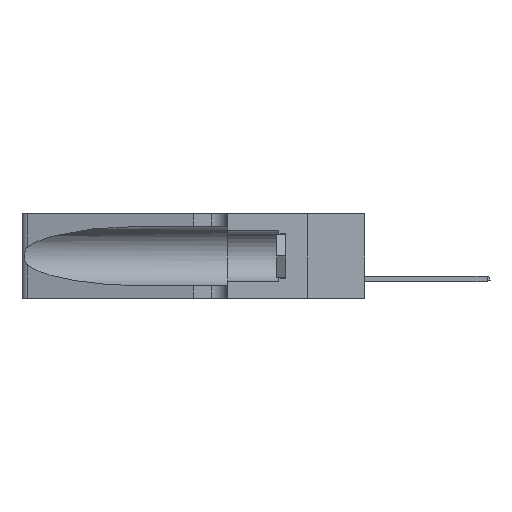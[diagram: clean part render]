
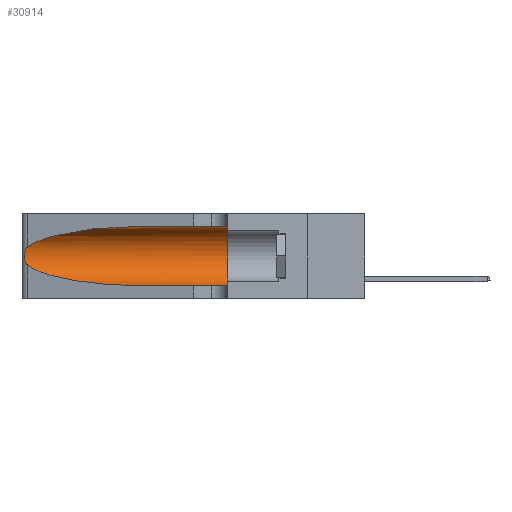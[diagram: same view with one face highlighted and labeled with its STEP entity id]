
A CAD part, left-side view. The second image highlights one B-rep face of the part: STEP entity #30914.
In plain terms, the highlighted cylindrical face has radius 3.308 mm (diameter 6.617 mm), a partial arc.
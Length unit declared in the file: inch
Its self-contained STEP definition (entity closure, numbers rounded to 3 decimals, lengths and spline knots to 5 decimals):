
#700 = CARTESIAN_POINT ( 'NONE',  ( 0.1305, 1.61858, 0.185 ) ) ;
#908 = CARTESIAN_POINT ( 'NONE',  ( 0.2373, 1.15595, 0.08982 ) ) ;
#1054 = ORIENTED_EDGE ( 'NONE', *, *, #3222, .T. ) ;
#1078 = CARTESIAN_POINT ( 'NONE',  ( 0.25487, 1.22718, 0.22369 ) ) ;
#1785 = CARTESIAN_POINT ( 'NONE',  ( 0.26017, 1.23833, 0.17102 ) ) ;
#2062 = CARTESIAN_POINT ( 'NONE',  ( 0.25555, 1.22993, 0.14849 ) ) ;
#3222 = EDGE_CURVE ( 'NONE', #4837, #20518, #38762, .T. ) ;
#4233 = DIRECTION ( 'NONE',  ( 0., -1., 0. ) ) ;
#4286 = CARTESIAN_POINT ( 'NONE',  ( 0.1305, 1.61858, 0.31525 ) ) ;
#4837 = VERTEX_POINT ( 'NONE', #37128 ) ;
#4975 = LINE ( 'NONE', #4286, #26247 ) ;
#5872 = ORIENTED_EDGE ( 'NONE', *, *, #35247, .F. ) ;
#5877 = FACE_OUTER_BOUND ( 'NONE', #23993, .T. ) ;
#6115 = AXIS2_PLACEMENT_3D ( 'NONE', #31212, #37541, #15209 ) ;
#6388 = ORIENTED_EDGE ( 'NONE', *, *, #33840, .F. ) ;
#6869 = CARTESIAN_POINT ( 'NONE',  ( 0.25487, 1.22718, 0.14631 ) ) ;
#7342 = CARTESIAN_POINT ( 'NONE',  ( 0.18966, 0.96281, 0.31525 ) ) ;
#7866 = VERTEX_POINT ( 'NONE', #13988 ) ;
#8295 = CARTESIAN_POINT ( 'NONE',  ( 0.25487, 1.22718, 0.14631 ) ) ;
#9068 = CARTESIAN_POINT ( 'NONE',  ( 0.1305, 0.72297, 0.31525 ) ) ;
#9539 = CARTESIAN_POINT ( 'NONE',  ( 0.1305, 0.35, 0.31525 ) ) ;
#9937 =( BOUNDED_CURVE ( )  B_SPLINE_CURVE ( 3, ( #9068, #7342, #10147, #1078 ),
 .UNSPECIFIED., .F., .F. ) 
 B_SPLINE_CURVE_WITH_KNOTS ( ( 4, 4 ),
 ( 1.5708, 2.84003 ),
 .UNSPECIFIED. ) 
 CURVE ( )  GEOMETRIC_REPRESENTATION_ITEM ( )  RATIONAL_B_SPLINE_CURVE ( ( 1., 0.87, 0.87, 1. ) ) 
 REPRESENTATION_ITEM ( '' )  );
#10120 = CARTESIAN_POINT ( 'NONE',  ( 0.18966, 0.96281, 0.05475 ) ) ;
#10147 = CARTESIAN_POINT ( 'NONE',  ( 0.2373, 1.15595, 0.28018 ) ) ;
#11411 = CARTESIAN_POINT ( 'NONE',  ( 0.25787, 1.23484, 0.2124 ) ) ;
#12643 = ORIENTED_EDGE ( 'NONE', *, *, #15343, .T. ) ;
#13561 = DIRECTION ( 'NONE',  ( 0., 0., -1. ) ) ;
#13988 = CARTESIAN_POINT ( 'NONE',  ( 0.1305, 0.72297, 0.31525 ) ) ;
#14921 = CARTESIAN_POINT ( 'NONE',  ( 0.25854, 1.2359, 0.20912 ) ) ;
#15205 = CARTESIAN_POINT ( 'NONE',  ( 0.26075, 1.23896, 0.178 ) ) ;
#15209 = DIRECTION ( 'NONE',  ( 0., 0., 1. ) ) ;
#15343 = EDGE_CURVE ( 'NONE', #7866, #41217, #9937, .T. ) ;
#20518 = VERTEX_POINT ( 'NONE', #26975 ) ;
#21016 = CARTESIAN_POINT ( 'NONE',  ( 0.25856, 1.23593, 0.16098 ) ) ;
#21431 = CARTESIAN_POINT ( 'NONE',  ( 0.25639, 1.23186, 0.15144 ) ) ;
#21580 = CARTESIAN_POINT ( 'NONE',  ( 0.25487, 1.22718, 0.22369 ) ) ;
#22164 = VERTEX_POINT ( 'NONE', #25880 ) ;
#23993 = EDGE_LOOP ( 'NONE', ( #12643, #41035, #24847, #1054, #5872, #6388 ) ) ;
#24411 = CARTESIAN_POINT ( 'NONE',  ( 0.25789, 1.23486, 0.15765 ) ) ;
#24847 = ORIENTED_EDGE ( 'NONE', *, *, #32039, .T. ) ;
#25765 = DIRECTION ( 'NONE',  ( 0., -1., 0. ) ) ;
#25880 = CARTESIAN_POINT ( 'NONE',  ( 0.25487, 1.22718, 0.14631 ) ) ;
#26092 = CARTESIAN_POINT ( 'NONE',  ( 0.1305, 0.72297, 0.05475 ) ) ;
#26247 = VECTOR ( 'NONE', #30467, 39.37008 ) ;
#26975 = CARTESIAN_POINT ( 'NONE',  ( 0.1305, 0.35, 0.05475 ) ) ;
#27406 =( BOUNDED_CURVE ( )  B_SPLINE_CURVE ( 3, ( #6869, #908, #10120, #26092 ),
 .UNSPECIFIED., .F., .F. ) 
 B_SPLINE_CURVE_WITH_KNOTS ( ( 4, 4 ),
 ( 3.44316, 4.71239 ),
 .UNSPECIFIED. ) 
 CURVE ( )  GEOMETRIC_REPRESENTATION_ITEM ( )  RATIONAL_B_SPLINE_CURVE ( ( 1., 0.87, 0.87, 1. ) ) 
 REPRESENTATION_ITEM ( '' )  );
#28104 = CARTESIAN_POINT ( 'NONE',  ( 0.25639, 1.23184, 0.21858 ) ) ;
#28592 = VERTEX_POINT ( 'NONE', #9539 ) ;
#29433 = CARTESIAN_POINT ( 'NONE',  ( 0.1305, 1.61858, 0.05475 ) ) ;
#29949 = EDGE_CURVE ( 'NONE', #41217, #22164, #34139, .T. ) ;
#30467 = DIRECTION ( 'NONE',  ( 0., -1., 0. ) ) ;
#30770 = CARTESIAN_POINT ( 'NONE',  ( 0.25487, 1.22718, 0.22369 ) ) ;
#30914 = ADVANCED_FACE ( 'NONE', ( #5877 ), #41683, .F. ) ;
#31212 = CARTESIAN_POINT ( 'NONE',  ( 0.1305, 0.35, 0.185 ) ) ;
#31336 = CARTESIAN_POINT ( 'NONE',  ( 0.26075, 1.23896, 0.19203 ) ) ;
#32039 = EDGE_CURVE ( 'NONE', #22164, #4837, #27406, .T. ) ;
#33186 = VECTOR ( 'NONE', #25765, 39.37008 ) ;
#33840 = EDGE_CURVE ( 'NONE', #7866, #28592, #4975, .T. ) ;
#34139 = B_SPLINE_CURVE_WITH_KNOTS ( 'NONE', 3,
 ( #21580, #34291, #28104, #11411, #14921, #40788, #31336, #15205, #1785, #21016, #24411, #21431, #2062, #8295 ),
 .UNSPECIFIED., .F., .F.,
 ( 4, 2, 2, 2, 2, 2, 4 ),
 ( 0., 0.00027, 0.00053, 0.00107, 0.0016, 0.00187, 0.00214 ),
 .UNSPECIFIED. ) ;
#34291 = CARTESIAN_POINT ( 'NONE',  ( 0.25555, 1.22994, 0.2215 ) ) ;
#35247 = EDGE_CURVE ( 'NONE', #28592, #20518, #38255, .T. ) ;
#37128 = CARTESIAN_POINT ( 'NONE',  ( 0.1305, 0.72297, 0.05475 ) ) ;
#37541 = DIRECTION ( 'NONE',  ( 0., 1., 0. ) ) ;
#38255 = CIRCLE ( 'NONE', #6115, 0.13025 ) ;
#38762 = LINE ( 'NONE', #29433, #33186 ) ;
#39539 = AXIS2_PLACEMENT_3D ( 'NONE', #700, #4233, #13561 ) ;
#40788 = CARTESIAN_POINT ( 'NONE',  ( 0.26018, 1.23835, 0.19895 ) ) ;
#41035 = ORIENTED_EDGE ( 'NONE', *, *, #29949, .T. ) ;
#41217 = VERTEX_POINT ( 'NONE', #30770 ) ;
#41683 = CYLINDRICAL_SURFACE ( 'NONE', #39539, 0.13025 ) ;
